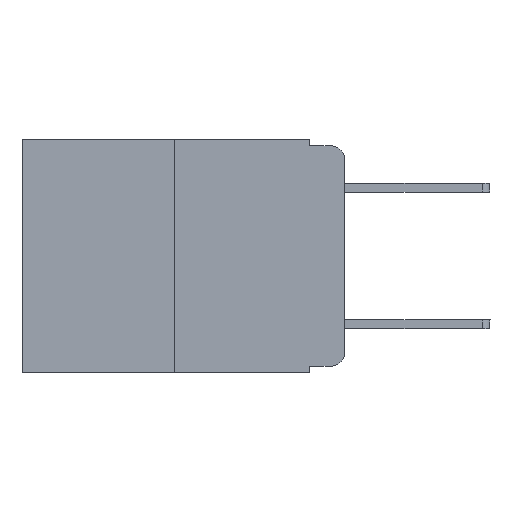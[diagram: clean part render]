
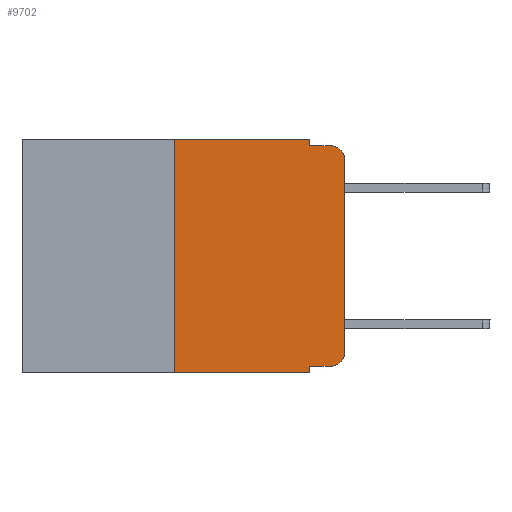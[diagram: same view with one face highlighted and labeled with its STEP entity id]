
A CAD part, left-side view. The second image highlights one B-rep face of the part: STEP entity #9702.
In plain terms, the highlighted planar face has unit normal (-1, 0, 0).
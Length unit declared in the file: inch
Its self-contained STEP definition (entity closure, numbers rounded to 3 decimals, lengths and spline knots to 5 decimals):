
#532 = LINE ( 'NONE', #14378, #6164 ) ;
#1206 = ORIENTED_EDGE ( 'NONE', *, *, #12997, .F. ) ;
#1326 = ORIENTED_EDGE ( 'NONE', *, *, #13250, .F. ) ;
#1427 = VERTEX_POINT ( 'NONE', #13268 ) ;
#1577 = EDGE_CURVE ( 'NONE', #12375, #15559, #2153, .T. ) ;
#2153 = LINE ( 'NONE', #11122, #3750 ) ;
#2268 = VECTOR ( 'NONE', #7759, 39.37008 ) ;
#2475 = VERTEX_POINT ( 'NONE', #5114 ) ;
#2601 = ORIENTED_EDGE ( 'NONE', *, *, #13541, .F. ) ;
#2956 = EDGE_CURVE ( 'NONE', #4602, #15478, #11569, .T. ) ;
#3145 = VECTOR ( 'NONE', #12468, 39.37008 ) ;
#3390 = DIRECTION ( 'NONE',  ( 0., 0., -1. ) ) ;
#3750 = VECTOR ( 'NONE', #3390, 39.37008 ) ;
#3925 = DIRECTION ( 'NONE',  ( 1., 0., 0. ) ) ;
#4288 = CARTESIAN_POINT ( 'NONE',  ( 0., 0.051, -0.343 ) ) ;
#4308 = VECTOR ( 'NONE', #13045, 39.37008 ) ;
#4494 = CARTESIAN_POINT ( 'NONE',  ( 0., 0.02, -0.313 ) ) ;
#4602 = VERTEX_POINT ( 'NONE', #8208 ) ;
#4675 = VECTOR ( 'NONE', #8641, 39.37008 ) ;
#4775 = ORIENTED_EDGE ( 'NONE', *, *, #2956, .T. ) ;
#5114 = CARTESIAN_POINT ( 'NONE',  ( 0., 0.02, -0.01 ) ) ;
#5574 = EDGE_CURVE ( 'NONE', #7134, #15559, #6584, .T. ) ;
#5721 = DIRECTION ( 'NONE',  ( 0., 0., -1. ) ) ;
#5890 = EDGE_CURVE ( 'NONE', #12375, #14898, #532, .T. ) ;
#6164 = VECTOR ( 'NONE', #7830, 39.37008 ) ;
#6453 = DIRECTION ( 'NONE',  ( 0., 0., -1. ) ) ;
#6584 = LINE ( 'NONE', #10079, #3145 ) ;
#6594 = CARTESIAN_POINT ( 'NONE',  ( 0., 0.25, 0. ) ) ;
#6795 = ORIENTED_EDGE ( 'NONE', *, *, #10109, .T. ) ;
#7084 = VERTEX_POINT ( 'NONE', #7795 ) ;
#7134 = VERTEX_POINT ( 'NONE', #15576 ) ;
#7526 = PLANE ( 'NONE',  #15136 ) ;
#7759 = DIRECTION ( 'NONE',  ( 0., -1., 0. ) ) ;
#7795 = CARTESIAN_POINT ( 'NONE',  ( 0., 0.051, 0. ) ) ;
#7830 = DIRECTION ( 'NONE',  ( 0., -1., 0. ) ) ;
#8021 = CARTESIAN_POINT ( 'NONE',  ( 0., 0.02, -0.333 ) ) ;
#8208 = CARTESIAN_POINT ( 'NONE',  ( 0., 0., -0.313 ) ) ;
#8347 = ORIENTED_EDGE ( 'NONE', *, *, #5574, .T. ) ;
#8403 = CARTESIAN_POINT ( 'NONE',  ( 0., 0.25, 0. ) ) ;
#8475 = DIRECTION ( 'NONE',  ( 0., 0., -1. ) ) ;
#8641 = DIRECTION ( 'NONE',  ( 0., 0., 1. ) ) ;
#8986 = EDGE_CURVE ( 'NONE', #15879, #7084, #11689, .T. ) ;
#9050 = CIRCLE ( 'NONE', #10201, 0.02 ) ;
#9259 = CIRCLE ( 'NONE', #14399, 0.02 ) ;
#9514 = EDGE_CURVE ( 'NONE', #15478, #2475, #9050, .T. ) ;
#9702 = ADVANCED_FACE ( 'NONE', ( #13235 ), #7526, .F. ) ;
#10079 = CARTESIAN_POINT ( 'NONE',  ( 0., 0.473, -0.343 ) ) ;
#10109 = EDGE_CURVE ( 'NONE', #14898, #4602, #9259, .T. ) ;
#10201 = AXIS2_PLACEMENT_3D ( 'NONE', #16126, #13574, #8475 ) ;
#11092 = LINE ( 'NONE', #8403, #4675 ) ;
#11122 = CARTESIAN_POINT ( 'NONE',  ( 0., 0.051, 0. ) ) ;
#11569 = LINE ( 'NONE', #12342, #16424 ) ;
#11641 = CARTESIAN_POINT ( 'NONE',  ( 0., 0., -0.03 ) ) ;
#11689 = LINE ( 'NONE', #13091, #2268 ) ;
#11696 = CARTESIAN_POINT ( 'NONE',  ( 0., 0.051, 0. ) ) ;
#12342 = CARTESIAN_POINT ( 'NONE',  ( 0., 0., 0. ) ) ;
#12375 = VERTEX_POINT ( 'NONE', #14905 ) ;
#12468 = DIRECTION ( 'NONE',  ( 0., -1., 0. ) ) ;
#12731 = LINE ( 'NONE', #14902, #13321 ) ;
#12810 = ORIENTED_EDGE ( 'NONE', *, *, #5890, .T. ) ;
#12997 = EDGE_CURVE ( 'NONE', #7084, #1427, #13747, .T. ) ;
#13045 = DIRECTION ( 'NONE',  ( 0., 0., -1. ) ) ;
#13091 = CARTESIAN_POINT ( 'NONE',  ( 0., 0.473, 0. ) ) ;
#13235 = FACE_OUTER_BOUND ( 'NONE', #15114, .T. ) ;
#13250 = EDGE_CURVE ( 'NONE', #1427, #2475, #12731, .T. ) ;
#13268 = CARTESIAN_POINT ( 'NONE',  ( 0., 0.051, -0.01 ) ) ;
#13321 = VECTOR ( 'NONE', #13428, 39.37008 ) ;
#13380 = ORIENTED_EDGE ( 'NONE', *, *, #8986, .F. ) ;
#13415 = DIRECTION ( 'NONE',  ( -1., 0., 0. ) ) ;
#13428 = DIRECTION ( 'NONE',  ( 0., -1., 0. ) ) ;
#13541 = EDGE_CURVE ( 'NONE', #7134, #15879, #11092, .T. ) ;
#13574 = DIRECTION ( 'NONE',  ( -1., 0., 0. ) ) ;
#13747 = LINE ( 'NONE', #11696, #4308 ) ;
#14378 = CARTESIAN_POINT ( 'NONE',  ( 0., 0.051, -0.333 ) ) ;
#14399 = AXIS2_PLACEMENT_3D ( 'NONE', #4494, #13415, #5721 ) ;
#14535 = ORIENTED_EDGE ( 'NONE', *, *, #9514, .T. ) ;
#14651 = ORIENTED_EDGE ( 'NONE', *, *, #1577, .F. ) ;
#14898 = VERTEX_POINT ( 'NONE', #8021 ) ;
#14902 = CARTESIAN_POINT ( 'NONE',  ( 0., 0.051, -0.01 ) ) ;
#14905 = CARTESIAN_POINT ( 'NONE',  ( 0., 0.051, -0.333 ) ) ;
#15114 = EDGE_LOOP ( 'NONE', ( #4775, #14535, #1326, #1206, #13380, #2601, #8347, #14651, #12810, #6795 ) ) ;
#15136 = AXIS2_PLACEMENT_3D ( 'NONE', #15319, #3925, #6453 ) ;
#15319 = CARTESIAN_POINT ( 'NONE',  ( 0., 0.473, 0. ) ) ;
#15478 = VERTEX_POINT ( 'NONE', #11641 ) ;
#15559 = VERTEX_POINT ( 'NONE', #4288 ) ;
#15576 = CARTESIAN_POINT ( 'NONE',  ( 0., 0.25, -0.343 ) ) ;
#15879 = VERTEX_POINT ( 'NONE', #6594 ) ;
#16126 = CARTESIAN_POINT ( 'NONE',  ( 0., 0.02, -0.03 ) ) ;
#16417 = DIRECTION ( 'NONE',  ( 0., 0., 1. ) ) ;
#16424 = VECTOR ( 'NONE', #16417, 39.37008 ) ;
